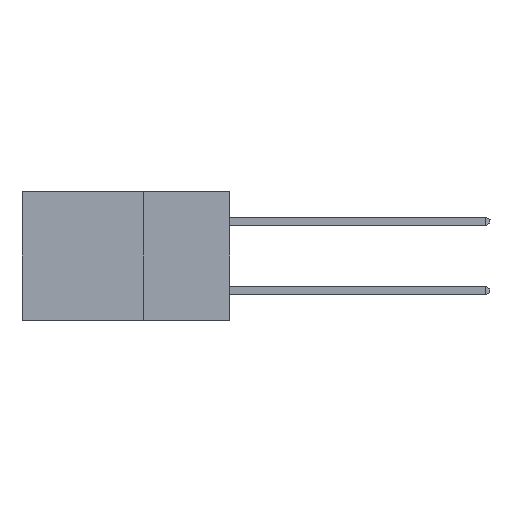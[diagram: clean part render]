
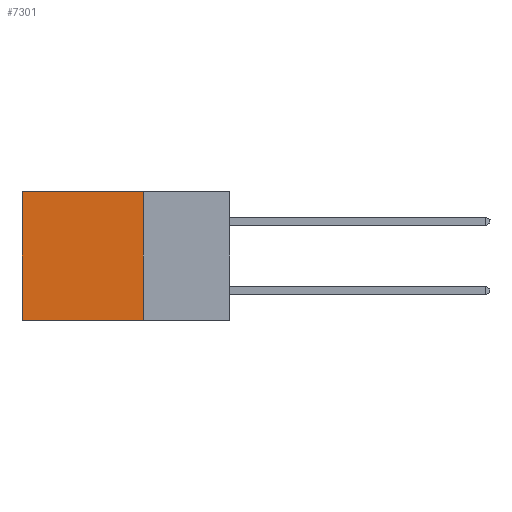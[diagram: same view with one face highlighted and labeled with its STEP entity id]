
A CAD part, left-side view. The second image highlights one B-rep face of the part: STEP entity #7301.
In plain terms, the highlighted planar face has unit normal (-1, 0, 0).
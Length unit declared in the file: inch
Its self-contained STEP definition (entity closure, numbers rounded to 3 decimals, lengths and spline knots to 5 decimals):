
#126 = DIRECTION ( 'NONE',  ( 0., 1., 0. ) ) ;
#2101 = VERTEX_POINT ( 'NONE', #3593 ) ;
#2421 = VECTOR ( 'NONE', #29734, 39.37008 ) ;
#3005 = VERTEX_POINT ( 'NONE', #32376 ) ;
#3428 = CARTESIAN_POINT ( 'NONE',  ( 0.298, 0.6, 0. ) ) ;
#3593 = CARTESIAN_POINT ( 'NONE',  ( 0.298, 0.25, -0.37 ) ) ;
#3599 = LINE ( 'NONE', #32250, #7924 ) ;
#6538 = AXIS2_PLACEMENT_3D ( 'NONE', #29636, #29527, #12176 ) ;
#7017 = CARTESIAN_POINT ( 'NONE',  ( 0.298, 0.6, 0. ) ) ;
#7301 = ADVANCED_FACE ( 'NONE', ( #18330 ), #22005, .F. ) ;
#7924 = VECTOR ( 'NONE', #17175, 39.37008 ) ;
#9074 = EDGE_CURVE ( 'NONE', #13211, #3005, #32394, .T. ) ;
#9791 = CARTESIAN_POINT ( 'NONE',  ( 0.298, 0.25, 0. ) ) ;
#10783 = VERTEX_POINT ( 'NONE', #27137 ) ;
#12176 = DIRECTION ( 'NONE',  ( 0., 0., -1. ) ) ;
#13211 = VERTEX_POINT ( 'NONE', #7017 ) ;
#15696 = EDGE_CURVE ( 'NONE', #10783, #2101, #3599, .T. ) ;
#16519 = EDGE_LOOP ( 'NONE', ( #18928, #17732, #24045, #19189 ) ) ;
#17175 = DIRECTION ( 'NONE',  ( 0., 0., -1. ) ) ;
#17732 = ORIENTED_EDGE ( 'NONE', *, *, #31179, .F. ) ;
#18330 = FACE_OUTER_BOUND ( 'NONE', #16519, .T. ) ;
#18928 = ORIENTED_EDGE ( 'NONE', *, *, #9074, .T. ) ;
#19189 = ORIENTED_EDGE ( 'NONE', *, *, #26296, .T. ) ;
#22005 = PLANE ( 'NONE',  #6538 ) ;
#22944 = VECTOR ( 'NONE', #29162, 39.37008 ) ;
#23156 = VECTOR ( 'NONE', #126, 39.37008 ) ;
#24045 = ORIENTED_EDGE ( 'NONE', *, *, #15696, .F. ) ;
#25135 = CARTESIAN_POINT ( 'NONE',  ( 0.298, 0.25, -0.37 ) ) ;
#25955 = LINE ( 'NONE', #25135, #2421 ) ;
#26296 = EDGE_CURVE ( 'NONE', #10783, #13211, #28230, .T. ) ;
#27137 = CARTESIAN_POINT ( 'NONE',  ( 0.298, 0.25, 0. ) ) ;
#28230 = LINE ( 'NONE', #9791, #23156 ) ;
#29162 = DIRECTION ( 'NONE',  ( 0., 0., -1. ) ) ;
#29527 = DIRECTION ( 'NONE',  ( 1., 0., 0. ) ) ;
#29636 = CARTESIAN_POINT ( 'NONE',  ( 0.298, 0.25, 0. ) ) ;
#29734 = DIRECTION ( 'NONE',  ( 0., 1., 0. ) ) ;
#31179 = EDGE_CURVE ( 'NONE', #2101, #3005, #25955, .T. ) ;
#32250 = CARTESIAN_POINT ( 'NONE',  ( 0.298, 0.25, 0. ) ) ;
#32376 = CARTESIAN_POINT ( 'NONE',  ( 0.298, 0.6, -0.37 ) ) ;
#32394 = LINE ( 'NONE', #3428, #22944 ) ;
